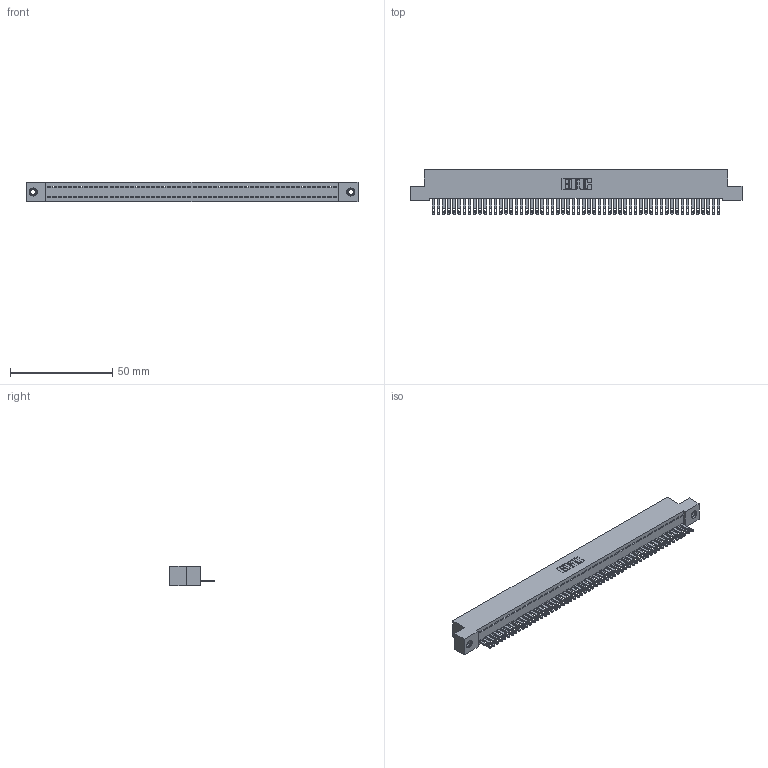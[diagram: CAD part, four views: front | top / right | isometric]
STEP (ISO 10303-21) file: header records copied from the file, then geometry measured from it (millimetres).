
FILE_DESCRIPTION (( 'STEP AP203' ), '1' );
FILE_NAME ('342-056-500-107.STEP', '2018-08-13T02:02:03', ( '' ), ( '' ), 'SwSTEP 2.0', 'SolidWorks 2016', '' );
FILE_SCHEMA (( 'CONFIG_CONTROL_DESIGN' ));
Length unit declared in the file: inch
Products named in the file (4): 342 Part_TI; 345-292-001_345-293-100; 345-250-001_345-250-005-103; 342-056-500-107
Assembly tree (59 placements, depth 2):
  342-056-500-107
    342 Part_TI
    345-292-001_345-293-100  x56
    345-250-001_345-250-005-103  x2
Bounding box: 162.56 x 21.85 x 9.4 mm (x, y, z)
Volume: 14326.8 mm3; surface area: 21442.1 mm2
Topology: 59 solids, 59 shells, 3194 faces, 9843 edges, 6554 vertices
Faces by surface type: plane 2114, cylinder 1064, cone 12, torus 4
Entity records: 33408 total; most frequent: CARTESIAN_POINT 5741, ORIENTED_EDGE 5726, DIRECTION 4849, EDGE_CURVE 2863, VECTOR 2711, LINE 2711, VERTEX_POINT 1904, AXIS2_PLACEMENT_3D 1069
